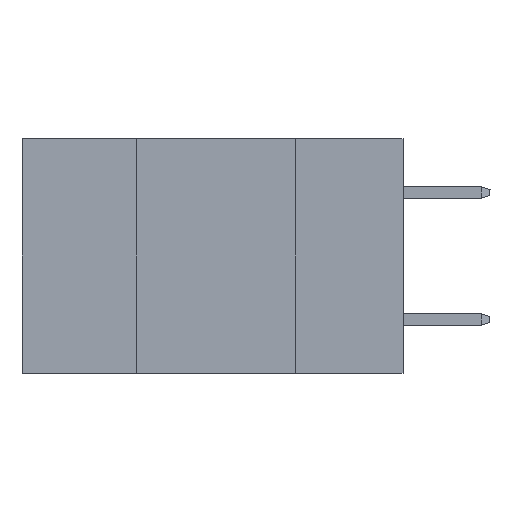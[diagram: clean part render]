
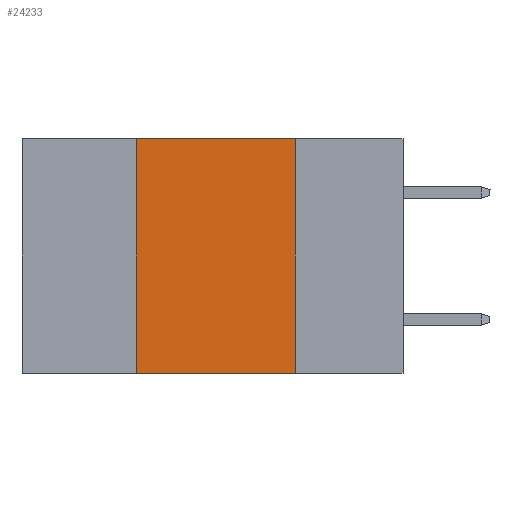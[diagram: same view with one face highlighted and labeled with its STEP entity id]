
A CAD part, left-side view. The second image highlights one B-rep face of the part: STEP entity #24233.
In plain terms, the highlighted planar face has unit normal (-1, 0, 0).
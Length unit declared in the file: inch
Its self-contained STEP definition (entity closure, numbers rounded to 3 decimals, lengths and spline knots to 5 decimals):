
#1196 = VERTEX_POINT ( 'NONE', #18676 ) ;
#1260 = FACE_OUTER_BOUND ( 'NONE', #8492, .T. ) ;
#1473 = PLANE ( 'NONE',  #8918 ) ;
#2598 = CARTESIAN_POINT ( 'NONE',  ( 0., 0.6, 0. ) ) ;
#4683 = EDGE_CURVE ( 'NONE', #8802, #1196, #36105, .T. ) ;
#5578 = EDGE_CURVE ( 'NONE', #22828, #8802, #8911, .T. ) ;
#7317 = CARTESIAN_POINT ( 'NONE',  ( 0., 0.6, 0. ) ) ;
#8492 = EDGE_LOOP ( 'NONE', ( #11242, #9367, #23030, #30808 ) ) ;
#8802 = VERTEX_POINT ( 'NONE', #25607 ) ;
#8911 = LINE ( 'NONE', #9808, #23270 ) ;
#8918 = AXIS2_PLACEMENT_3D ( 'NONE', #7317, #17816, #15115 ) ;
#9367 = ORIENTED_EDGE ( 'NONE', *, *, #4683, .F. ) ;
#9808 = CARTESIAN_POINT ( 'NONE',  ( 0., 0.42, 0. ) ) ;
#11014 = CARTESIAN_POINT ( 'NONE',  ( 0., 0.17, -0.37 ) ) ;
#11242 = ORIENTED_EDGE ( 'NONE', *, *, #13482, .F. ) ;
#13482 = EDGE_CURVE ( 'NONE', #1196, #18752, #22610, .T. ) ;
#15115 = DIRECTION ( 'NONE',  ( 0., 0., -1. ) ) ;
#16052 = DIRECTION ( 'NONE',  ( 0., 0., 1. ) ) ;
#16160 = VECTOR ( 'NONE', #19470, 39.37008 ) ;
#16217 = DIRECTION ( 'NONE',  ( 0., -1., 0. ) ) ;
#17041 = LINE ( 'NONE', #17250, #39623 ) ;
#17250 = CARTESIAN_POINT ( 'NONE',  ( 0., 0.6, -0.37 ) ) ;
#17816 = DIRECTION ( 'NONE',  ( 1., 0., 0. ) ) ;
#18676 = CARTESIAN_POINT ( 'NONE',  ( 0., 0.17, 0. ) ) ;
#18752 = VERTEX_POINT ( 'NONE', #11014 ) ;
#19470 = DIRECTION ( 'NONE',  ( 0., 0., -1. ) ) ;
#22610 = LINE ( 'NONE', #26189, #16160 ) ;
#22828 = VERTEX_POINT ( 'NONE', #41485 ) ;
#23030 = ORIENTED_EDGE ( 'NONE', *, *, #5578, .F. ) ;
#23270 = VECTOR ( 'NONE', #16052, 39.37008 ) ;
#23985 = DIRECTION ( 'NONE',  ( 0., -1., 0. ) ) ;
#24233 = ADVANCED_FACE ( 'NONE', ( #1260 ), #1473, .F. ) ;
#25607 = CARTESIAN_POINT ( 'NONE',  ( 0., 0.42, 0. ) ) ;
#26189 = CARTESIAN_POINT ( 'NONE',  ( 0., 0.17, 0. ) ) ;
#30223 = EDGE_CURVE ( 'NONE', #22828, #18752, #17041, .T. ) ;
#30808 = ORIENTED_EDGE ( 'NONE', *, *, #30223, .T. ) ;
#33856 = VECTOR ( 'NONE', #16217, 39.37008 ) ;
#36105 = LINE ( 'NONE', #2598, #33856 ) ;
#39623 = VECTOR ( 'NONE', #23985, 39.37008 ) ;
#41485 = CARTESIAN_POINT ( 'NONE',  ( 0., 0.42, -0.37 ) ) ;
